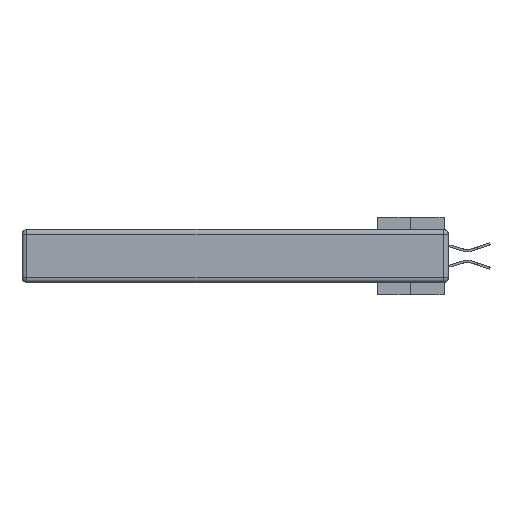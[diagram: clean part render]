
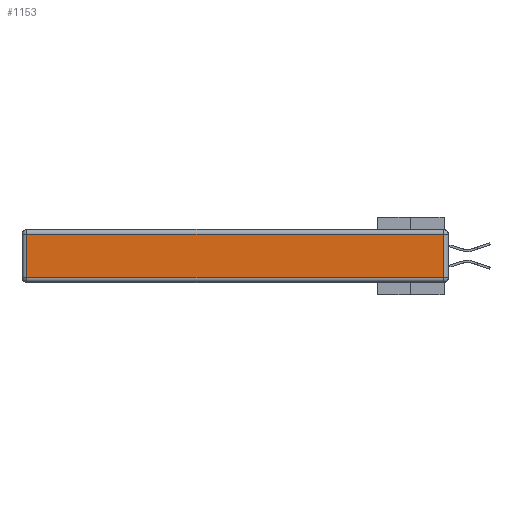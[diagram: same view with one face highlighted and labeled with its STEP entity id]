
A CAD part, left-side view. The second image highlights one B-rep face of the part: STEP entity #1153.
In plain terms, the highlighted planar face has unit normal (-1, 0, 0).
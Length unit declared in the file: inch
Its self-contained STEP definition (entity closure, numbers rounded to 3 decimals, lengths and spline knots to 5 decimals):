
#19 = CARTESIAN_POINT ( 'NONE',  ( 0., 0.03, -0.03 ) ) ;
#450 = LINE ( 'NONE', #10517, #14301 ) ;
#670 = EDGE_CURVE ( 'NONE', #14271, #19272, #8612, .T. ) ;
#1153 = ADVANCED_FACE ( 'NONE', ( #31607 ), #21515, .T. ) ;
#1430 = CARTESIAN_POINT ( 'NONE',  ( 0., 2.75, -0.03 ) ) ;
#2467 = EDGE_CURVE ( 'NONE', #9417, #16633, #450, .T. ) ;
#2937 = CARTESIAN_POINT ( 'NONE',  ( 0., 0.03, -0.313 ) ) ;
#7645 = DIRECTION ( 'NONE',  ( -1., 0., 0. ) ) ;
#8612 = LINE ( 'NONE', #37101, #10817 ) ;
#9417 = VERTEX_POINT ( 'NONE', #21013 ) ;
#9917 = ORIENTED_EDGE ( 'NONE', *, *, #670, .T. ) ;
#10517 = CARTESIAN_POINT ( 'NONE',  ( 0., 2.72, -0.343 ) ) ;
#10817 = VECTOR ( 'NONE', #16351, 39.37008 ) ;
#12008 = AXIS2_PLACEMENT_3D ( 'NONE', #30247, #7645, #15928 ) ;
#14271 = VERTEX_POINT ( 'NONE', #2937 ) ;
#14301 = VECTOR ( 'NONE', #16936, 39.37008 ) ;
#14534 = DIRECTION ( 'NONE',  ( 0., -1., 0. ) ) ;
#15928 = DIRECTION ( 'NONE',  ( 0., 0., 1. ) ) ;
#16351 = DIRECTION ( 'NONE',  ( 0., 0., 1. ) ) ;
#16633 = VERTEX_POINT ( 'NONE', #22464 ) ;
#16936 = DIRECTION ( 'NONE',  ( 0., 0., -1. ) ) ;
#17644 = LINE ( 'NONE', #1430, #19469 ) ;
#19272 = VERTEX_POINT ( 'NONE', #19 ) ;
#19469 = VECTOR ( 'NONE', #32811, 39.37008 ) ;
#19829 = VECTOR ( 'NONE', #14534, 39.37008 ) ;
#21013 = CARTESIAN_POINT ( 'NONE',  ( 0., 2.72, -0.03 ) ) ;
#21515 = PLANE ( 'NONE',  #12008 ) ;
#22464 = CARTESIAN_POINT ( 'NONE',  ( 0., 2.72, -0.313 ) ) ;
#22488 = ORIENTED_EDGE ( 'NONE', *, *, #28274, .T. ) ;
#23166 = CARTESIAN_POINT ( 'NONE',  ( 0., 0., -0.313 ) ) ;
#25274 = LINE ( 'NONE', #23166, #19829 ) ;
#26026 = EDGE_LOOP ( 'NONE', ( #36698, #9917, #22488, #27139 ) ) ;
#27139 = ORIENTED_EDGE ( 'NONE', *, *, #2467, .T. ) ;
#28274 = EDGE_CURVE ( 'NONE', #19272, #9417, #17644, .T. ) ;
#30247 = CARTESIAN_POINT ( 'NONE',  ( 0., 0., -0.343 ) ) ;
#31607 = FACE_OUTER_BOUND ( 'NONE', #26026, .T. ) ;
#32811 = DIRECTION ( 'NONE',  ( 0., 1., 0. ) ) ;
#36119 = EDGE_CURVE ( 'NONE', #16633, #14271, #25274, .T. ) ;
#36698 = ORIENTED_EDGE ( 'NONE', *, *, #36119, .T. ) ;
#37101 = CARTESIAN_POINT ( 'NONE',  ( 0., 0.03, -0.343 ) ) ;
